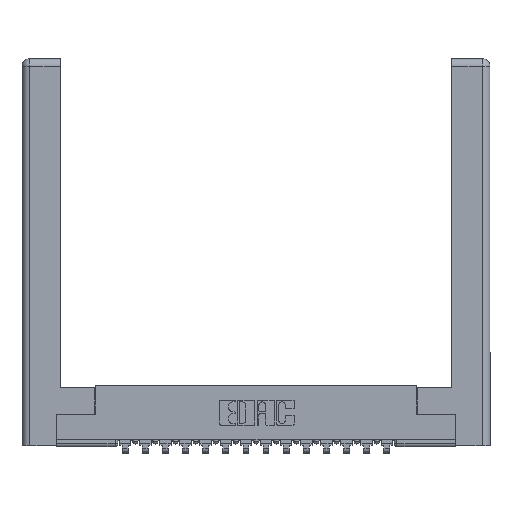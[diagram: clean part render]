
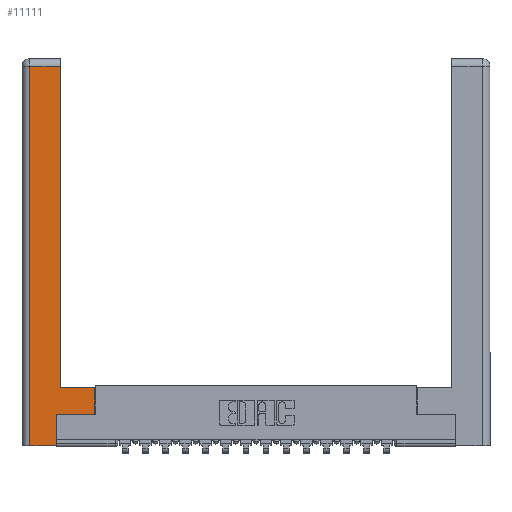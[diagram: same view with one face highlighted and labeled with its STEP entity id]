
A CAD part, top view. The second image highlights one B-rep face of the part: STEP entity #11111.
In plain terms, the highlighted planar face has unit normal (0, 0, 1).
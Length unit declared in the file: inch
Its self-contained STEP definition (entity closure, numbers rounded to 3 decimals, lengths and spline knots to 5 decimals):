
#133 = CARTESIAN_POINT ( 'NONE',  ( 0.0615, 2.94, 0. ) ) ;
#357 = VECTOR ( 'NONE', #13711, 39.37008 ) ;
#787 = LINE ( 'NONE', #14039, #17195 ) ;
#1454 = VERTEX_POINT ( 'NONE', #15757 ) ;
#1486 = VERTEX_POINT ( 'NONE', #4135 ) ;
#1680 = AXIS2_PLACEMENT_3D ( 'NONE', #9476, #2198, #2383 ) ;
#2198 = DIRECTION ( 'NONE',  ( 0., 0., -1. ) ) ;
#2237 = EDGE_CURVE ( 'NONE', #10625, #6908, #18197, .T. ) ;
#2383 = DIRECTION ( 'NONE',  ( -1., 0., 0. ) ) ;
#2581 = CARTESIAN_POINT ( 'NONE',  ( 0.295, 0.45, 0. ) ) ;
#3219 = ORIENTED_EDGE ( 'NONE', *, *, #17728, .T. ) ;
#3346 = LINE ( 'NONE', #11994, #7518 ) ;
#3383 = DIRECTION ( 'NONE',  ( -1., 0., 0. ) ) ;
#3615 = DIRECTION ( 'NONE',  ( 0., 1., 0. ) ) ;
#3796 = EDGE_CURVE ( 'NONE', #13694, #14767, #9253, .T. ) ;
#3820 = ORIENTED_EDGE ( 'NONE', *, *, #7514, .T. ) ;
#3845 = DIRECTION ( 'NONE',  ( 1., 0., 0. ) ) ;
#4135 = CARTESIAN_POINT ( 'NONE',  ( 0.265, 0., 0. ) ) ;
#5032 = ORIENTED_EDGE ( 'NONE', *, *, #2237, .T. ) ;
#5254 = VERTEX_POINT ( 'NONE', #5976 ) ;
#5375 = EDGE_CURVE ( 'NONE', #1454, #13694, #6353, .T. ) ;
#5421 = CARTESIAN_POINT ( 'NONE',  ( 0.295, 3., 0. ) ) ;
#5947 = EDGE_CURVE ( 'NONE', #14767, #14196, #18574, .T. ) ;
#5976 = CARTESIAN_POINT ( 'NONE',  ( 0.295, 2.94, 0. ) ) ;
#6353 = LINE ( 'NONE', #9426, #12894 ) ;
#6680 = FACE_OUTER_BOUND ( 'NONE', #7792, .T. ) ;
#6908 = VERTEX_POINT ( 'NONE', #11711 ) ;
#7514 = EDGE_CURVE ( 'NONE', #14196, #5254, #15616, .T. ) ;
#7518 = VECTOR ( 'NONE', #7757, 39.37008 ) ;
#7577 = VECTOR ( 'NONE', #14373, 39.37008 ) ;
#7603 = DIRECTION ( 'NONE',  ( 1., 0., 0. ) ) ;
#7757 = DIRECTION ( 'NONE',  ( 0., 1., 0. ) ) ;
#7792 = EDGE_LOOP ( 'NONE', ( #3820, #9914, #5032, #3219, #11773, #15594, #11061, #10532 ) ) ;
#7831 = CARTESIAN_POINT ( 'NONE',  ( 0.0615, 0., 0. ) ) ;
#8505 = CARTESIAN_POINT ( 'NONE',  ( 0.295, 0.45, 0. ) ) ;
#9061 = DIRECTION ( 'NONE',  ( 0., 1., 0. ) ) ;
#9253 = LINE ( 'NONE', #15121, #9528 ) ;
#9426 = CARTESIAN_POINT ( 'NONE',  ( 0.565, 0.245, 0. ) ) ;
#9476 = CARTESIAN_POINT ( 'NONE',  ( 0., 0., 0. ) ) ;
#9528 = VECTOR ( 'NONE', #9061, 39.37008 ) ;
#9657 = EDGE_CURVE ( 'NONE', #5254, #10625, #15011, .T. ) ;
#9914 = ORIENTED_EDGE ( 'NONE', *, *, #9657, .T. ) ;
#10532 = ORIENTED_EDGE ( 'NONE', *, *, #5947, .T. ) ;
#10625 = VERTEX_POINT ( 'NONE', #11831 ) ;
#11061 = ORIENTED_EDGE ( 'NONE', *, *, #3796, .T. ) ;
#11111 = ADVANCED_FACE ( 'NONE', ( #6680 ), #12547, .F. ) ;
#11711 = CARTESIAN_POINT ( 'NONE',  ( 0.0615, 0., 0. ) ) ;
#11773 = ORIENTED_EDGE ( 'NONE', *, *, #13926, .T. ) ;
#11831 = CARTESIAN_POINT ( 'NONE',  ( 0.0615, 2.94, 0. ) ) ;
#11994 = CARTESIAN_POINT ( 'NONE',  ( 0.265, 0.245, 0. ) ) ;
#12022 = CARTESIAN_POINT ( 'NONE',  ( 0.565, 0.45, 0. ) ) ;
#12547 = PLANE ( 'NONE',  #1680 ) ;
#12680 = CARTESIAN_POINT ( 'NONE',  ( 0.565, 0.245, 0. ) ) ;
#12894 = VECTOR ( 'NONE', #7603, 39.37008 ) ;
#13213 = VECTOR ( 'NONE', #3615, 39.37008 ) ;
#13694 = VERTEX_POINT ( 'NONE', #12680 ) ;
#13711 = DIRECTION ( 'NONE',  ( 0., -1., 0. ) ) ;
#13926 = EDGE_CURVE ( 'NONE', #1486, #1454, #3346, .T. ) ;
#14039 = CARTESIAN_POINT ( 'NONE',  ( 0.265, 0., 0. ) ) ;
#14196 = VERTEX_POINT ( 'NONE', #2581 ) ;
#14204 = VECTOR ( 'NONE', #3383, 39.37008 ) ;
#14373 = DIRECTION ( 'NONE',  ( -1., 0., 0. ) ) ;
#14767 = VERTEX_POINT ( 'NONE', #12022 ) ;
#15011 = LINE ( 'NONE', #133, #14204 ) ;
#15121 = CARTESIAN_POINT ( 'NONE',  ( 0.565, 0.45, 0. ) ) ;
#15594 = ORIENTED_EDGE ( 'NONE', *, *, #5375, .T. ) ;
#15616 = LINE ( 'NONE', #5421, #13213 ) ;
#15757 = CARTESIAN_POINT ( 'NONE',  ( 0.265, 0.245, 0. ) ) ;
#17195 = VECTOR ( 'NONE', #3845, 39.37008 ) ;
#17728 = EDGE_CURVE ( 'NONE', #6908, #1486, #787, .T. ) ;
#18197 = LINE ( 'NONE', #7831, #357 ) ;
#18574 = LINE ( 'NONE', #8505, #7577 ) ;
